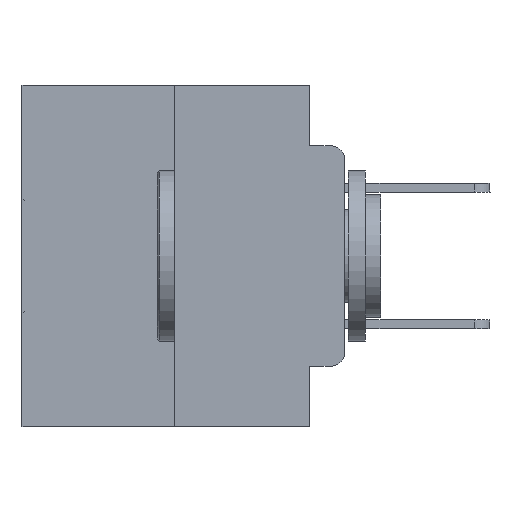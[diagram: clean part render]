
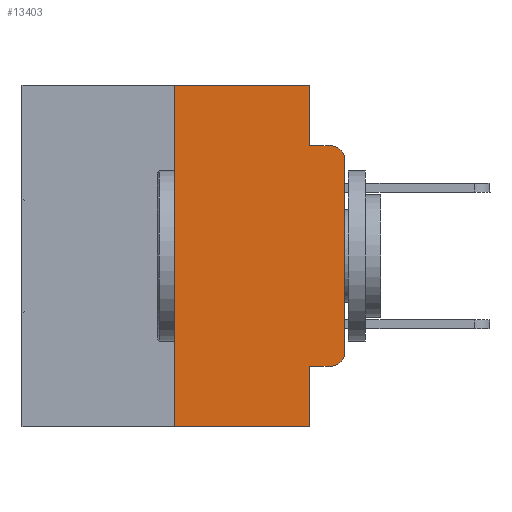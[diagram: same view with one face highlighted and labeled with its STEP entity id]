
A CAD part, left-side view. The second image highlights one B-rep face of the part: STEP entity #13403.
In plain terms, the highlighted planar face has unit normal (-1, 0, 0).
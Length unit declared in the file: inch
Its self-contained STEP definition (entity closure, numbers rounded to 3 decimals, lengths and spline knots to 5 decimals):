
#78 = VECTOR ( 'NONE', #15215, 39.37008 ) ;
#265 = VERTEX_POINT ( 'NONE', #22626 ) ;
#432 = VERTEX_POINT ( 'NONE', #16954 ) ;
#541 = DIRECTION ( 'NONE',  ( 0., 0., -1. ) ) ;
#1187 = CARTESIAN_POINT ( 'NONE',  ( 0., 0.051, -0.4115 ) ) ;
#1248 = LINE ( 'NONE', #3216, #15311 ) ;
#1797 = CARTESIAN_POINT ( 'NONE',  ( 0., 0.25, 0. ) ) ;
#2145 = EDGE_CURVE ( 'NONE', #15947, #24632, #7909, .T. ) ;
#2727 = PLANE ( 'NONE',  #4252 ) ;
#2813 = VERTEX_POINT ( 'NONE', #16199 ) ;
#2830 = EDGE_CURVE ( 'NONE', #15610, #4435, #21611, .T. ) ;
#3216 = CARTESIAN_POINT ( 'NONE',  ( 0., 0.051, -0.0885 ) ) ;
#3358 = EDGE_CURVE ( 'NONE', #432, #23175, #16267, .T. ) ;
#3425 = CARTESIAN_POINT ( 'NONE',  ( 0., 0.051, 0. ) ) ;
#4252 = AXIS2_PLACEMENT_3D ( 'NONE', #14768, #26790, #17321 ) ;
#4400 = AXIS2_PLACEMENT_3D ( 'NONE', #5634, #7658, #541 ) ;
#4435 = VERTEX_POINT ( 'NONE', #5122 ) ;
#4790 = CARTESIAN_POINT ( 'NONE',  ( 0., 0., 0. ) ) ;
#5024 = AXIS2_PLACEMENT_3D ( 'NONE', #23510, #14262, #9153 ) ;
#5122 = CARTESIAN_POINT ( 'NONE',  ( 0., 0.02, -0.0885 ) ) ;
#5314 = LINE ( 'NONE', #4790, #10244 ) ;
#5553 = VECTOR ( 'NONE', #20947, 39.37008 ) ;
#5634 = CARTESIAN_POINT ( 'NONE',  ( 0., 0.02, -0.3915 ) ) ;
#6247 = ORIENTED_EDGE ( 'NONE', *, *, #14579, .T. ) ;
#6361 = EDGE_LOOP ( 'NONE', ( #6247, #28046, #6536, #10726, #23404, #22773, #11620, #9813, #18936, #29103 ) ) ;
#6536 = ORIENTED_EDGE ( 'NONE', *, *, #25547, .F. ) ;
#6803 = LINE ( 'NONE', #10651, #29664 ) ;
#6851 = VERTEX_POINT ( 'NONE', #23181 ) ;
#7658 = DIRECTION ( 'NONE',  ( -1., 0., 0. ) ) ;
#7659 = CIRCLE ( 'NONE', #4400, 0.02 ) ;
#7889 = CARTESIAN_POINT ( 'NONE',  ( 0., 0.473, 0. ) ) ;
#7909 = LINE ( 'NONE', #29971, #22756 ) ;
#8072 = LINE ( 'NONE', #7889, #78 ) ;
#9153 = DIRECTION ( 'NONE',  ( 0., 0., -1. ) ) ;
#9584 = EDGE_CURVE ( 'NONE', #25615, #6851, #31410, .T. ) ;
#9761 = VECTOR ( 'NONE', #15444, 39.37008 ) ;
#9813 = ORIENTED_EDGE ( 'NONE', *, *, #27360, .F. ) ;
#10244 = VECTOR ( 'NONE', #24275, 39.37008 ) ;
#10490 = LINE ( 'NONE', #28002, #5553 ) ;
#10651 = CARTESIAN_POINT ( 'NONE',  ( 0., 0.051, 0. ) ) ;
#10726 = ORIENTED_EDGE ( 'NONE', *, *, #9584, .F. ) ;
#11328 = CARTESIAN_POINT ( 'NONE',  ( 0., 0.02, -0.4115 ) ) ;
#11620 = ORIENTED_EDGE ( 'NONE', *, *, #17581, .T. ) ;
#13403 = ADVANCED_FACE ( 'NONE', ( #15983 ), #2727, .F. ) ;
#14262 = DIRECTION ( 'NONE',  ( -1., 0., 0. ) ) ;
#14579 = EDGE_CURVE ( 'NONE', #265, #15610, #5314, .T. ) ;
#14768 = CARTESIAN_POINT ( 'NONE',  ( 0., 0.473, 0. ) ) ;
#15215 = DIRECTION ( 'NONE',  ( 0., -1., 0. ) ) ;
#15311 = VECTOR ( 'NONE', #20129, 39.37008 ) ;
#15444 = DIRECTION ( 'NONE',  ( 0., -1., 0. ) ) ;
#15610 = VERTEX_POINT ( 'NONE', #21336 ) ;
#15947 = VERTEX_POINT ( 'NONE', #20251 ) ;
#15983 = FACE_OUTER_BOUND ( 'NONE', #6361, .T. ) ;
#16199 = CARTESIAN_POINT ( 'NONE',  ( 0., 0.051, -0.5 ) ) ;
#16267 = LINE ( 'NONE', #1187, #9761 ) ;
#16954 = CARTESIAN_POINT ( 'NONE',  ( 0., 0.051, -0.4115 ) ) ;
#17236 = DIRECTION ( 'NONE',  ( 0., 0., -1. ) ) ;
#17321 = DIRECTION ( 'NONE',  ( 0., 0., -1. ) ) ;
#17581 = EDGE_CURVE ( 'NONE', #15947, #2813, #10490, .T. ) ;
#18936 = ORIENTED_EDGE ( 'NONE', *, *, #3358, .T. ) ;
#19962 = EDGE_CURVE ( 'NONE', #24632, #25615, #8072, .T. ) ;
#20025 = EDGE_CURVE ( 'NONE', #23175, #265, #7659, .T. ) ;
#20129 = DIRECTION ( 'NONE',  ( 0., -1., 0. ) ) ;
#20251 = CARTESIAN_POINT ( 'NONE',  ( 0., 0.25, -0.5 ) ) ;
#20947 = DIRECTION ( 'NONE',  ( 0., -1., 0. ) ) ;
#21336 = CARTESIAN_POINT ( 'NONE',  ( 0., 0., -0.1085 ) ) ;
#21611 = CIRCLE ( 'NONE', #5024, 0.02 ) ;
#22240 = CARTESIAN_POINT ( 'NONE',  ( 0., 0.051, 0. ) ) ;
#22626 = CARTESIAN_POINT ( 'NONE',  ( 0., 0., -0.3915 ) ) ;
#22756 = VECTOR ( 'NONE', #29758, 39.37008 ) ;
#22773 = ORIENTED_EDGE ( 'NONE', *, *, #2145, .F. ) ;
#23175 = VERTEX_POINT ( 'NONE', #11328 ) ;
#23181 = CARTESIAN_POINT ( 'NONE',  ( 0., 0.051, -0.0885 ) ) ;
#23404 = ORIENTED_EDGE ( 'NONE', *, *, #19962, .F. ) ;
#23510 = CARTESIAN_POINT ( 'NONE',  ( 0., 0.02, -0.1085 ) ) ;
#24275 = DIRECTION ( 'NONE',  ( 0., 0., 1. ) ) ;
#24632 = VERTEX_POINT ( 'NONE', #1797 ) ;
#24944 = VECTOR ( 'NONE', #17236, 39.37008 ) ;
#25547 = EDGE_CURVE ( 'NONE', #6851, #4435, #1248, .T. ) ;
#25615 = VERTEX_POINT ( 'NONE', #3425 ) ;
#26790 = DIRECTION ( 'NONE',  ( 1., 0., 0. ) ) ;
#27360 = EDGE_CURVE ( 'NONE', #432, #2813, #6803, .T. ) ;
#27708 = DIRECTION ( 'NONE',  ( 0., 0., -1. ) ) ;
#28002 = CARTESIAN_POINT ( 'NONE',  ( 0., 0.473, -0.5 ) ) ;
#28046 = ORIENTED_EDGE ( 'NONE', *, *, #2830, .T. ) ;
#29103 = ORIENTED_EDGE ( 'NONE', *, *, #20025, .T. ) ;
#29664 = VECTOR ( 'NONE', #27708, 39.37008 ) ;
#29758 = DIRECTION ( 'NONE',  ( 0., 0., 1. ) ) ;
#29971 = CARTESIAN_POINT ( 'NONE',  ( 0., 0.25, 0. ) ) ;
#31410 = LINE ( 'NONE', #22240, #24944 ) ;
